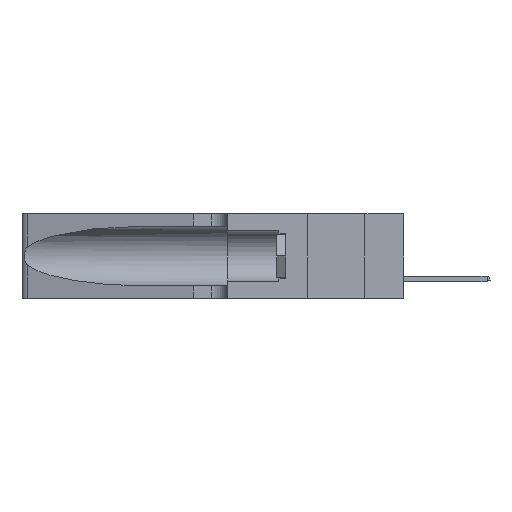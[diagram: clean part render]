
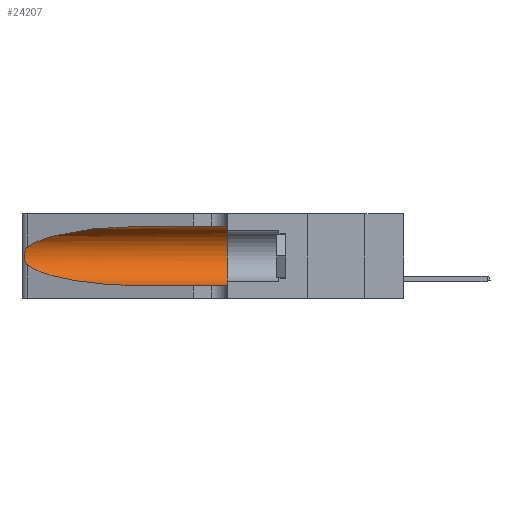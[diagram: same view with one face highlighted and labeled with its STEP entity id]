
A CAD part, left-side view. The second image highlights one B-rep face of the part: STEP entity #24207.
In plain terms, the highlighted cylindrical face has radius 3.308 mm (diameter 6.617 mm), a partial arc.
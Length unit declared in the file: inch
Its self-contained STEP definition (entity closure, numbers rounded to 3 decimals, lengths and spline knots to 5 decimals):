
#676 = B_SPLINE_CURVE_WITH_KNOTS ( 'NONE', 3,
 ( #39891, #17452, #27173, #33111, #16880, #20590, #23808, #31211, #36080, #16633, #27860, #4006, #9198, #31935 ),
 .UNSPECIFIED., .F., .F.,
 ( 4, 2, 2, 2, 2, 2, 4 ),
 ( 0., 0.00027, 0.00053, 0.00107, 0.0016, 0.00187, 0.00214 ),
 .UNSPECIFIED. ) ;
#1206 = ORIENTED_EDGE ( 'NONE', *, *, #21812, .F. ) ;
#2239 = DIRECTION ( 'NONE',  ( 0., 1., 0. ) ) ;
#2296 = VERTEX_POINT ( 'NONE', #6299 ) ;
#2478 = CARTESIAN_POINT ( 'NONE',  ( 0.25487, 1.22718, 0.14631 ) ) ;
#3039 = LINE ( 'NONE', #23093, #17727 ) ;
#3728 = DIRECTION ( 'NONE',  ( 0., -1., 0. ) ) ;
#3740 = EDGE_CURVE ( 'NONE', #10393, #16723, #3039, .T. ) ;
#4006 = CARTESIAN_POINT ( 'NONE',  ( 0.25639, 1.23186, 0.15144 ) ) ;
#5039 = CARTESIAN_POINT ( 'NONE',  ( 0.25487, 1.22718, 0.22369 ) ) ;
#5164 = CARTESIAN_POINT ( 'NONE',  ( 0.18966, 0.96281, 0.05475 ) ) ;
#5522 = DIRECTION ( 'NONE',  ( 0., 0., 1. ) ) ;
#6299 = CARTESIAN_POINT ( 'NONE',  ( 0.1305, 0.35, 0.05475 ) ) ;
#6351 = ORIENTED_EDGE ( 'NONE', *, *, #19033, .T. ) ;
#6848 = EDGE_LOOP ( 'NONE', ( #41941, #6351, #35987, #14613, #1206, #7544 ) ) ;
#6955 = DIRECTION ( 'NONE',  ( 0., -1., 0. ) ) ;
#7544 = ORIENTED_EDGE ( 'NONE', *, *, #3740, .F. ) ;
#7667 = AXIS2_PLACEMENT_3D ( 'NONE', #21510, #2239, #5522 ) ;
#9198 = CARTESIAN_POINT ( 'NONE',  ( 0.25555, 1.22993, 0.14849 ) ) ;
#10393 = VERTEX_POINT ( 'NONE', #18718 ) ;
#10902 = DIRECTION ( 'NONE',  ( 0., -1., 0. ) ) ;
#11351 = CARTESIAN_POINT ( 'NONE',  ( 0.1305, 0.72297, 0.05475 ) ) ;
#12703 = AXIS2_PLACEMENT_3D ( 'NONE', #41029, #3728, #39897 ) ;
#13068 = LINE ( 'NONE', #30235, #19662 ) ;
#14613 = ORIENTED_EDGE ( 'NONE', *, *, #38807, .T. ) ;
#15935 = CYLINDRICAL_SURFACE ( 'NONE', #12703, 0.13025 ) ;
#16204 = CARTESIAN_POINT ( 'NONE',  ( 0.25487, 1.22718, 0.14631 ) ) ;
#16633 = CARTESIAN_POINT ( 'NONE',  ( 0.25856, 1.23593, 0.16098 ) ) ;
#16723 = VERTEX_POINT ( 'NONE', #17514 ) ;
#16880 = CARTESIAN_POINT ( 'NONE',  ( 0.25854, 1.2359, 0.20912 ) ) ;
#16944 = VERTEX_POINT ( 'NONE', #16204 ) ;
#17452 = CARTESIAN_POINT ( 'NONE',  ( 0.25555, 1.22994, 0.2215 ) ) ;
#17514 = CARTESIAN_POINT ( 'NONE',  ( 0.1305, 0.35, 0.31525 ) ) ;
#17727 = VECTOR ( 'NONE', #6955, 39.37008 ) ;
#17886 =( BOUNDED_CURVE ( )  B_SPLINE_CURVE ( 3, ( #31192, #18089, #28086, #5039 ),
 .UNSPECIFIED., .F., .F. ) 
 B_SPLINE_CURVE_WITH_KNOTS ( ( 4, 4 ),
 ( 1.5708, 2.84003 ),
 .UNSPECIFIED. ) 
 CURVE ( )  GEOMETRIC_REPRESENTATION_ITEM ( )  RATIONAL_B_SPLINE_CURVE ( ( 1., 0.87, 0.87, 1. ) ) 
 REPRESENTATION_ITEM ( '' )  );
#18089 = CARTESIAN_POINT ( 'NONE',  ( 0.18966, 0.96281, 0.31525 ) ) ;
#18718 = CARTESIAN_POINT ( 'NONE',  ( 0.1305, 0.72297, 0.31525 ) ) ;
#19033 = EDGE_CURVE ( 'NONE', #34425, #16944, #676, .T. ) ;
#19662 = VECTOR ( 'NONE', #10902, 39.37008 ) ;
#20590 = CARTESIAN_POINT ( 'NONE',  ( 0.26018, 1.23835, 0.19895 ) ) ;
#21459 = EDGE_CURVE ( 'NONE', #10393, #34425, #17886, .T. ) ;
#21510 = CARTESIAN_POINT ( 'NONE',  ( 0.1305, 0.35, 0.185 ) ) ;
#21812 = EDGE_CURVE ( 'NONE', #16723, #2296, #32676, .T. ) ;
#23003 = EDGE_CURVE ( 'NONE', #16944, #29973, #29547, .T. ) ;
#23093 = CARTESIAN_POINT ( 'NONE',  ( 0.1305, 1.61858, 0.31525 ) ) ;
#23808 = CARTESIAN_POINT ( 'NONE',  ( 0.26075, 1.23896, 0.19203 ) ) ;
#24207 = ADVANCED_FACE ( 'NONE', ( #29532 ), #15935, .F. ) ;
#27173 = CARTESIAN_POINT ( 'NONE',  ( 0.25639, 1.23184, 0.21858 ) ) ;
#27860 = CARTESIAN_POINT ( 'NONE',  ( 0.25789, 1.23486, 0.15765 ) ) ;
#28086 = CARTESIAN_POINT ( 'NONE',  ( 0.2373, 1.15595, 0.28018 ) ) ;
#29532 = FACE_OUTER_BOUND ( 'NONE', #6848, .T. ) ;
#29547 =( BOUNDED_CURVE ( )  B_SPLINE_CURVE ( 3, ( #2478, #31612, #5164, #40632 ),
 .UNSPECIFIED., .F., .F. ) 
 B_SPLINE_CURVE_WITH_KNOTS ( ( 4, 4 ),
 ( 3.44316, 4.71239 ),
 .UNSPECIFIED. ) 
 CURVE ( )  GEOMETRIC_REPRESENTATION_ITEM ( )  RATIONAL_B_SPLINE_CURVE ( ( 1., 0.87, 0.87, 1. ) ) 
 REPRESENTATION_ITEM ( '' )  );
#29973 = VERTEX_POINT ( 'NONE', #11351 ) ;
#30235 = CARTESIAN_POINT ( 'NONE',  ( 0.1305, 1.61858, 0.05475 ) ) ;
#31192 = CARTESIAN_POINT ( 'NONE',  ( 0.1305, 0.72297, 0.31525 ) ) ;
#31211 = CARTESIAN_POINT ( 'NONE',  ( 0.26075, 1.23896, 0.178 ) ) ;
#31612 = CARTESIAN_POINT ( 'NONE',  ( 0.2373, 1.15595, 0.08982 ) ) ;
#31935 = CARTESIAN_POINT ( 'NONE',  ( 0.25487, 1.22718, 0.14631 ) ) ;
#32676 = CIRCLE ( 'NONE', #7667, 0.13025 ) ;
#33111 = CARTESIAN_POINT ( 'NONE',  ( 0.25787, 1.23484, 0.2124 ) ) ;
#34425 = VERTEX_POINT ( 'NONE', #38310 ) ;
#35987 = ORIENTED_EDGE ( 'NONE', *, *, #23003, .T. ) ;
#36080 = CARTESIAN_POINT ( 'NONE',  ( 0.26017, 1.23833, 0.17102 ) ) ;
#38310 = CARTESIAN_POINT ( 'NONE',  ( 0.25487, 1.22718, 0.22369 ) ) ;
#38807 = EDGE_CURVE ( 'NONE', #29973, #2296, #13068, .T. ) ;
#39891 = CARTESIAN_POINT ( 'NONE',  ( 0.25487, 1.22718, 0.22369 ) ) ;
#39897 = DIRECTION ( 'NONE',  ( 0., 0., -1. ) ) ;
#40632 = CARTESIAN_POINT ( 'NONE',  ( 0.1305, 0.72297, 0.05475 ) ) ;
#41029 = CARTESIAN_POINT ( 'NONE',  ( 0.1305, 1.61858, 0.185 ) ) ;
#41941 = ORIENTED_EDGE ( 'NONE', *, *, #21459, .T. ) ;
